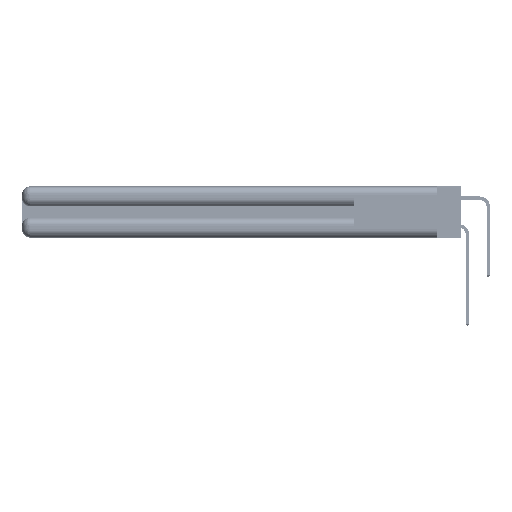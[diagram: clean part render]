
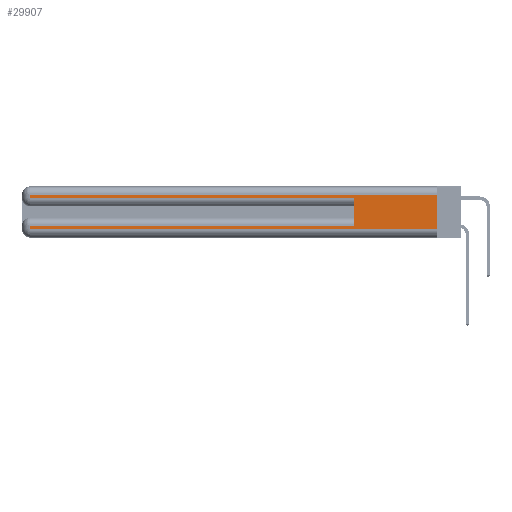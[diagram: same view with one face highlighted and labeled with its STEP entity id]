
A CAD part, left-side view. The second image highlights one B-rep face of the part: STEP entity #29907.
In plain terms, the highlighted planar face has unit normal (-1, 0, 0).
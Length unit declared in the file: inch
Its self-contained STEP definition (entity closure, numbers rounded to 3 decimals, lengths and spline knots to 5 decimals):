
#91 = EDGE_CURVE ( 'NONE', #23322, #19703, #175, .T. ) ;
#175 = LINE ( 'NONE', #33799, #12151 ) ;
#508 = ORIENTED_EDGE ( 'NONE', *, *, #24130, .F. ) ;
#592 = AXIS2_PLACEMENT_3D ( 'NONE', #3127, #47244, #23099 ) ;
#1974 = DIRECTION ( 'NONE',  ( 0., 0., 1. ) ) ;
#3127 = CARTESIAN_POINT ( 'NONE',  ( 0., 0., 0.37 ) ) ;
#3729 = DIRECTION ( 'NONE',  ( 0., -1., 0. ) ) ;
#4934 = CARTESIAN_POINT ( 'NONE',  ( 0., 0.6, 0.085 ) ) ;
#5300 = VERTEX_POINT ( 'NONE', #34385 ) ;
#6097 = VECTOR ( 'NONE', #9095, 39.37008 ) ;
#6204 = CARTESIAN_POINT ( 'NONE',  ( 0., 0.6, 0.145 ) ) ;
#6355 = CARTESIAN_POINT ( 'NONE',  ( 0., 0., 0.285 ) ) ;
#6502 = DIRECTION ( 'NONE',  ( 0., 0., -1. ) ) ;
#7718 = EDGE_CURVE ( 'NONE', #51763, #43169, #32585, .T. ) ;
#8844 = VECTOR ( 'NONE', #39221, 39.37008 ) ;
#9094 = VECTOR ( 'NONE', #3729, 39.37008 ) ;
#9095 = DIRECTION ( 'NONE',  ( 0., 1., 0. ) ) ;
#9271 = CARTESIAN_POINT ( 'NONE',  ( 0., 0., 0.085 ) ) ;
#9905 = DIRECTION ( 'NONE',  ( 0., -1., 0. ) ) ;
#11122 = EDGE_LOOP ( 'NONE', ( #14620, #48515, #42412, #25976, #508, #12390, #37484, #44509 ) ) ;
#11756 = CARTESIAN_POINT ( 'NONE',  ( 0., 2.94, 0.31 ) ) ;
#12082 = VERTEX_POINT ( 'NONE', #4934 ) ;
#12151 = VECTOR ( 'NONE', #47357, 39.37008 ) ;
#12390 = ORIENTED_EDGE ( 'NONE', *, *, #40492, .T. ) ;
#12981 = DIRECTION ( 'NONE',  ( 0., 0., -1. ) ) ;
#13001 = EDGE_CURVE ( 'NONE', #43169, #49573, #27693, .T. ) ;
#14419 = LINE ( 'NONE', #6204, #49152 ) ;
#14541 = VECTOR ( 'NONE', #12981, 39.37008 ) ;
#14620 = ORIENTED_EDGE ( 'NONE', *, *, #91, .F. ) ;
#16189 = LINE ( 'NONE', #9271, #6097 ) ;
#19277 = CARTESIAN_POINT ( 'NONE',  ( 0., 0., 0.31 ) ) ;
#19703 = VERTEX_POINT ( 'NONE', #39929 ) ;
#19773 = CARTESIAN_POINT ( 'NONE',  ( 0., 0., 0.06 ) ) ;
#20376 = CARTESIAN_POINT ( 'NONE',  ( 0., 0., 0.31 ) ) ;
#21708 = CARTESIAN_POINT ( 'NONE',  ( 0., 2.94, 0.37 ) ) ;
#23099 = DIRECTION ( 'NONE',  ( 0., 0., -1. ) ) ;
#23322 = VERTEX_POINT ( 'NONE', #20376 ) ;
#24130 = EDGE_CURVE ( 'NONE', #12082, #49573, #14419, .T. ) ;
#25976 = ORIENTED_EDGE ( 'NONE', *, *, #13001, .T. ) ;
#26205 = VERTEX_POINT ( 'NONE', #43809 ) ;
#26299 = EDGE_CURVE ( 'NONE', #26205, #19703, #32434, .T. ) ;
#26897 = VECTOR ( 'NONE', #6502, 39.37008 ) ;
#27693 = LINE ( 'NONE', #6355, #42876 ) ;
#27976 = EDGE_CURVE ( 'NONE', #23322, #51763, #43592, .T. ) ;
#29111 = CARTESIAN_POINT ( 'NONE',  ( 0., 0.6, 0.285 ) ) ;
#29746 = FACE_OUTER_BOUND ( 'NONE', #11122, .T. ) ;
#29907 = ADVANCED_FACE ( 'NONE', ( #29746 ), #38782, .F. ) ;
#32434 = LINE ( 'NONE', #19773, #9094 ) ;
#32585 = LINE ( 'NONE', #21708, #26897 ) ;
#33799 = CARTESIAN_POINT ( 'NONE',  ( 0., 0., 0.37 ) ) ;
#34385 = CARTESIAN_POINT ( 'NONE',  ( 0., 2.94, 0.085 ) ) ;
#36921 = CARTESIAN_POINT ( 'NONE',  ( 0., 2.94, 0.285 ) ) ;
#37484 = ORIENTED_EDGE ( 'NONE', *, *, #38482, .T. ) ;
#38482 = EDGE_CURVE ( 'NONE', #5300, #26205, #51175, .T. ) ;
#38782 = PLANE ( 'NONE',  #592 ) ;
#39221 = DIRECTION ( 'NONE',  ( 0., 1., 0. ) ) ;
#39929 = CARTESIAN_POINT ( 'NONE',  ( 0., 0., 0.06 ) ) ;
#40492 = EDGE_CURVE ( 'NONE', #12082, #5300, #16189, .T. ) ;
#42412 = ORIENTED_EDGE ( 'NONE', *, *, #7718, .T. ) ;
#42876 = VECTOR ( 'NONE', #9905, 39.37008 ) ;
#43169 = VERTEX_POINT ( 'NONE', #36921 ) ;
#43592 = LINE ( 'NONE', #19277, #8844 ) ;
#43809 = CARTESIAN_POINT ( 'NONE',  ( 0., 2.94, 0.06 ) ) ;
#44509 = ORIENTED_EDGE ( 'NONE', *, *, #26299, .T. ) ;
#47244 = DIRECTION ( 'NONE',  ( 1., 0., 0. ) ) ;
#47357 = DIRECTION ( 'NONE',  ( 0., 0., -1. ) ) ;
#48515 = ORIENTED_EDGE ( 'NONE', *, *, #27976, .T. ) ;
#48995 = CARTESIAN_POINT ( 'NONE',  ( 0., 2.94, 0.37 ) ) ;
#49152 = VECTOR ( 'NONE', #1974, 39.37008 ) ;
#49573 = VERTEX_POINT ( 'NONE', #29111 ) ;
#51175 = LINE ( 'NONE', #48995, #14541 ) ;
#51763 = VERTEX_POINT ( 'NONE', #11756 ) ;
